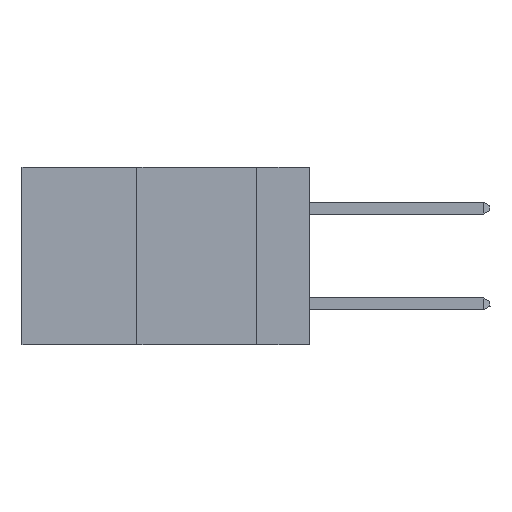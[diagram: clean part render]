
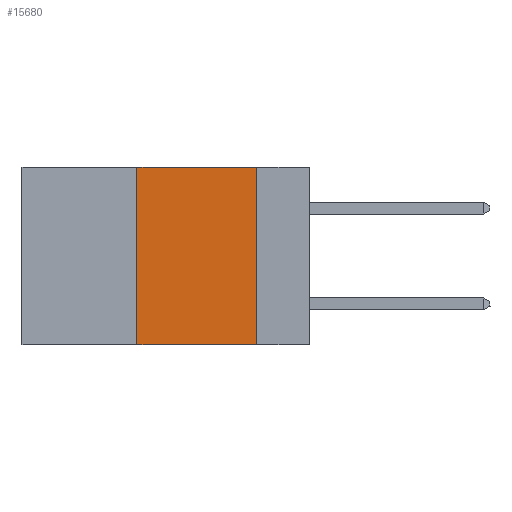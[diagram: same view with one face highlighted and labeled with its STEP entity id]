
A CAD part, left-side view. The second image highlights one B-rep face of the part: STEP entity #15680.
In plain terms, the highlighted planar face has unit normal (-1, 0, 0).
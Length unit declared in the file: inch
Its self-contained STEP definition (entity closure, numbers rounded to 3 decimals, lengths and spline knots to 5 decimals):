
#168 = PLANE ( 'NONE',  #20228 ) ;
#2327 = DIRECTION ( 'NONE',  ( 0., -1., 0. ) ) ;
#2427 = CARTESIAN_POINT ( 'NONE',  ( 0., 0.36, 0. ) ) ;
#2484 = CARTESIAN_POINT ( 'NONE',  ( 0., 0.36, -0.37 ) ) ;
#3133 = EDGE_CURVE ( 'NONE', #3651, #11437, #18798, .T. ) ;
#3632 = DIRECTION ( 'NONE',  ( 1., 0., 0. ) ) ;
#3651 = VERTEX_POINT ( 'NONE', #5284 ) ;
#4146 = DIRECTION ( 'NONE',  ( 0., 0., 1. ) ) ;
#4804 = DIRECTION ( 'NONE',  ( 0., 0., -1. ) ) ;
#4960 = CARTESIAN_POINT ( 'NONE',  ( 0., 0.11, 0. ) ) ;
#5181 = VECTOR ( 'NONE', #10452, 39.37008 ) ;
#5241 = VERTEX_POINT ( 'NONE', #5575 ) ;
#5284 = CARTESIAN_POINT ( 'NONE',  ( 0., 0.11, 0. ) ) ;
#5374 = LINE ( 'NONE', #2427, #10464 ) ;
#5575 = CARTESIAN_POINT ( 'NONE',  ( 0., 0.36, 0. ) ) ;
#9767 = EDGE_LOOP ( 'NONE', ( #10532, #11050, #16839, #18333 ) ) ;
#9994 = FACE_OUTER_BOUND ( 'NONE', #9767, .T. ) ;
#10169 = CARTESIAN_POINT ( 'NONE',  ( 0., 0.11, -0.37 ) ) ;
#10418 = EDGE_CURVE ( 'NONE', #19995, #5241, #5374, .T. ) ;
#10452 = DIRECTION ( 'NONE',  ( 0., -1., 0. ) ) ;
#10464 = VECTOR ( 'NONE', #4146, 39.37008 ) ;
#10532 = ORIENTED_EDGE ( 'NONE', *, *, #3133, .F. ) ;
#11050 = ORIENTED_EDGE ( 'NONE', *, *, #14508, .F. ) ;
#11437 = VERTEX_POINT ( 'NONE', #10169 ) ;
#11924 = VECTOR ( 'NONE', #2327, 39.37008 ) ;
#12002 = VECTOR ( 'NONE', #4804, 39.37008 ) ;
#13880 = CARTESIAN_POINT ( 'NONE',  ( 0., 0.6, 0. ) ) ;
#13907 = CARTESIAN_POINT ( 'NONE',  ( 0., 0.6, -0.37 ) ) ;
#14231 = CARTESIAN_POINT ( 'NONE',  ( 0., 0.6, 0. ) ) ;
#14508 = EDGE_CURVE ( 'NONE', #5241, #3651, #20994, .T. ) ;
#15029 = EDGE_CURVE ( 'NONE', #19995, #11437, #19361, .T. ) ;
#15594 = DIRECTION ( 'NONE',  ( 0., 0., -1. ) ) ;
#15680 = ADVANCED_FACE ( 'NONE', ( #9994 ), #168, .F. ) ;
#16839 = ORIENTED_EDGE ( 'NONE', *, *, #10418, .F. ) ;
#18333 = ORIENTED_EDGE ( 'NONE', *, *, #15029, .T. ) ;
#18798 = LINE ( 'NONE', #4960, #12002 ) ;
#19361 = LINE ( 'NONE', #13907, #5181 ) ;
#19995 = VERTEX_POINT ( 'NONE', #2484 ) ;
#20228 = AXIS2_PLACEMENT_3D ( 'NONE', #13880, #3632, #15594 ) ;
#20994 = LINE ( 'NONE', #14231, #11924 ) ;
